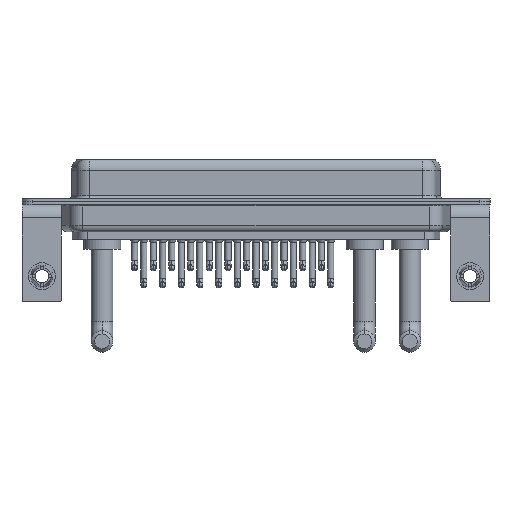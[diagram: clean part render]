
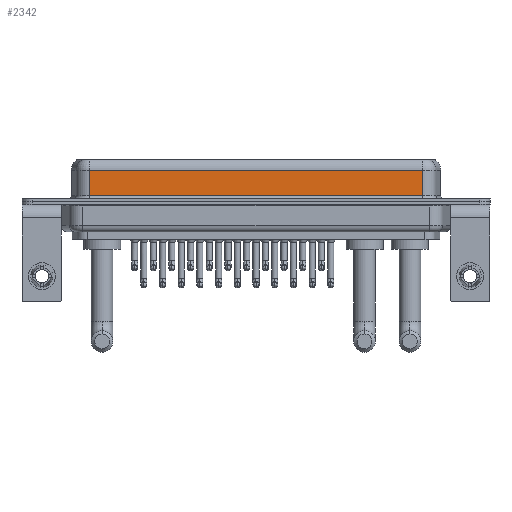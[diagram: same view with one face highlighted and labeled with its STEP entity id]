
A CAD part, front view. The second image highlights one B-rep face of the part: STEP entity #2342.
In plain terms, the highlighted planar face has unit normal (0, -1, 0).
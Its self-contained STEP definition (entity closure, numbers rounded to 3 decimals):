
#612 = LINE ( 'NONE', #2495, #18866 ) ;
#1480 = VERTEX_POINT ( 'NONE', #15889 ) ;
#2342 = ADVANCED_FACE ( 'NONE', ( #17545 ), #3453, .F. ) ;
#2495 = CARTESIAN_POINT ( 'NONE',  ( 56.462, -3.95, 0.9 ) ) ;
#2825 = ORIENTED_EDGE ( 'NONE', *, *, #6076, .T. ) ;
#3453 = PLANE ( 'NONE',  #22609 ) ;
#5430 = ORIENTED_EDGE ( 'NONE', *, *, #24986, .T. ) ;
#6076 = EDGE_CURVE ( 'NONE', #25874, #12932, #17755, .T. ) ;
#6470 = DIRECTION ( 'NONE',  ( 1., 0., 0. ) ) ;
#6501 = LINE ( 'NONE', #14607, #7007 ) ;
#6561 = DIRECTION ( 'NONE',  ( 0., 0., -1. ) ) ;
#7007 = VECTOR ( 'NONE', #22678, 1000. ) ;
#7932 = CARTESIAN_POINT ( 'NONE',  ( 56.462, -3.95, 4.65 ) ) ;
#7981 = VECTOR ( 'NONE', #9532, 1000. ) ;
#9532 = DIRECTION ( 'NONE',  ( -1., 0., 0. ) ) ;
#11245 = VERTEX_POINT ( 'NONE', #24574 ) ;
#11718 = CARTESIAN_POINT ( 'NONE',  ( 56.462, -3.95, 6.4 ) ) ;
#12500 = VECTOR ( 'NONE', #6561, 1000. ) ;
#12932 = VERTEX_POINT ( 'NONE', #14635 ) ;
#13353 = ORIENTED_EDGE ( 'NONE', *, *, #19861, .T. ) ;
#14524 = EDGE_LOOP ( 'NONE', ( #23435, #2825, #5430, #13353 ) ) ;
#14607 = CARTESIAN_POINT ( 'NONE',  ( 7.038, -3.95, 6.4 ) ) ;
#14635 = CARTESIAN_POINT ( 'NONE',  ( 7.038, -3.95, 4.65 ) ) ;
#14893 = CARTESIAN_POINT ( 'NONE',  ( 56.462, -3.95, 4.65 ) ) ;
#15889 = CARTESIAN_POINT ( 'NONE',  ( 7.038, -3.95, 0.9 ) ) ;
#16644 = LINE ( 'NONE', #24713, #12500 ) ;
#17545 = FACE_OUTER_BOUND ( 'NONE', #14524, .T. ) ;
#17755 = LINE ( 'NONE', #7932, #7981 ) ;
#17795 = EDGE_CURVE ( 'NONE', #25874, #11245, #16644, .T. ) ;
#18866 = VECTOR ( 'NONE', #6470, 1000. ) ;
#19861 = EDGE_CURVE ( 'NONE', #1480, #11245, #612, .T. ) ;
#21384 = DIRECTION ( 'NONE',  ( 0., 0., 1. ) ) ;
#22609 = AXIS2_PLACEMENT_3D ( 'NONE', #11718, #23499, #21384 ) ;
#22678 = DIRECTION ( 'NONE',  ( 0., 0., -1. ) ) ;
#23435 = ORIENTED_EDGE ( 'NONE', *, *, #17795, .F. ) ;
#23499 = DIRECTION ( 'NONE',  ( 0., 1., 0. ) ) ;
#24574 = CARTESIAN_POINT ( 'NONE',  ( 56.462, -3.95, 0.9 ) ) ;
#24713 = CARTESIAN_POINT ( 'NONE',  ( 56.462, -3.95, 6.4 ) ) ;
#24986 = EDGE_CURVE ( 'NONE', #12932, #1480, #6501, .T. ) ;
#25874 = VERTEX_POINT ( 'NONE', #14893 ) ;
